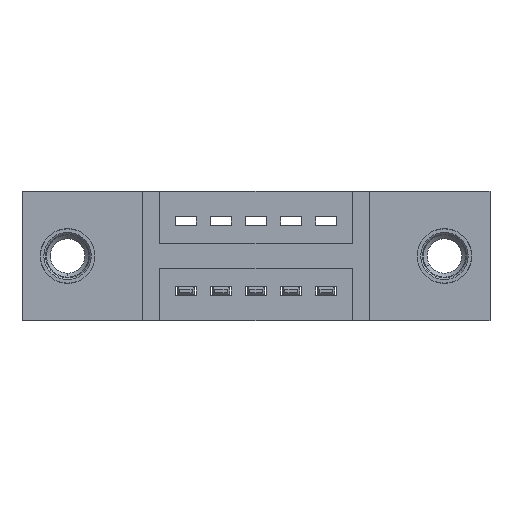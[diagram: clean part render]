
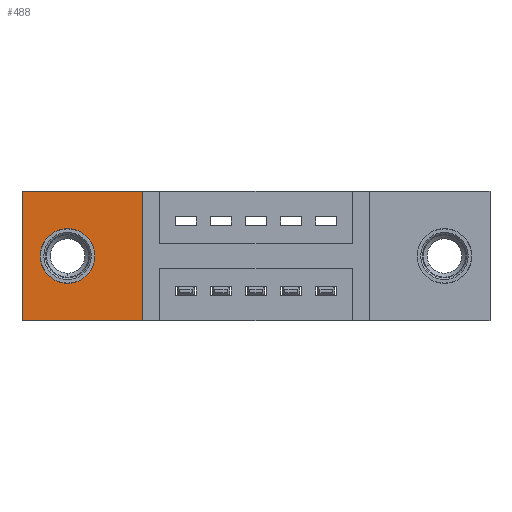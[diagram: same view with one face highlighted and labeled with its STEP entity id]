
A CAD part, front view. The second image highlights one B-rep face of the part: STEP entity #488.
In plain terms, the highlighted planar face has unit normal (0, -1, 0).
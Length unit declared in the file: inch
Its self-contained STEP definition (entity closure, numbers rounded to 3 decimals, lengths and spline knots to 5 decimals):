
#442 = FACE_BOUND ( 'NONE', #9706, .T. ) ;
#488 = ADVANCED_FACE ( 'NONE', ( #442, #2954 ), #3875, .T. ) ;
#566 = LINE ( 'NONE', #5035, #8496 ) ;
#1081 = AXIS2_PLACEMENT_3D ( 'NONE', #4815, #9822, #5535 ) ;
#1098 = CARTESIAN_POINT ( 'NONE',  ( 0.3425, 0.11, -0.37 ) ) ;
#1114 = ORIENTED_EDGE ( 'NONE', *, *, #1237, .T. ) ;
#1181 = CARTESIAN_POINT ( 'NONE',  ( 0.13, 0.11, -0.185 ) ) ;
#1237 = EDGE_CURVE ( 'NONE', #7051, #9205, #566, .T. ) ;
#1371 = EDGE_CURVE ( 'NONE', #5738, #6197, #5918, .T. ) ;
#1994 = DIRECTION ( 'NONE',  ( 0., 0., -1. ) ) ;
#2058 = DIRECTION ( 'NONE',  ( 0., 0., -1. ) ) ;
#2172 = CARTESIAN_POINT ( 'NONE',  ( 0., 0.11, 0. ) ) ;
#2687 = DIRECTION ( 'NONE',  ( 1., 0., 0. ) ) ;
#2844 = EDGE_CURVE ( 'NONE', #2900, #3693, #3410, .T. ) ;
#2900 = VERTEX_POINT ( 'NONE', #3859 ) ;
#2954 = FACE_OUTER_BOUND ( 'NONE', #9757, .T. ) ;
#3065 = DIRECTION ( 'NONE',  ( 0., -1., 0. ) ) ;
#3233 = CARTESIAN_POINT ( 'NONE',  ( 0.13, 0.11, -0.263 ) ) ;
#3410 = LINE ( 'NONE', #2172, #5218 ) ;
#3693 = VERTEX_POINT ( 'NONE', #6074 ) ;
#3859 = CARTESIAN_POINT ( 'NONE',  ( 0.3425, 0.11, 0. ) ) ;
#3875 = PLANE ( 'NONE',  #9088 ) ;
#4003 = CARTESIAN_POINT ( 'NONE',  ( 0., 0.11, -0.37 ) ) ;
#4101 = ORIENTED_EDGE ( 'NONE', *, *, #1371, .F. ) ;
#4141 = CARTESIAN_POINT ( 'NONE',  ( 0., 0.11, 0. ) ) ;
#4257 = VECTOR ( 'NONE', #6540, 39.37008 ) ;
#4375 = CARTESIAN_POINT ( 'NONE',  ( 0.3425, 0.11, 0. ) ) ;
#4726 = AXIS2_PLACEMENT_3D ( 'NONE', #1181, #6629, #2058 ) ;
#4815 = CARTESIAN_POINT ( 'NONE',  ( 0.13, 0.11, -0.185 ) ) ;
#5035 = CARTESIAN_POINT ( 'NONE',  ( 0., 0.11, -0.37 ) ) ;
#5188 = EDGE_CURVE ( 'NONE', #3693, #7051, #6234, .T. ) ;
#5218 = VECTOR ( 'NONE', #8172, 39.37008 ) ;
#5535 = DIRECTION ( 'NONE',  ( 0., 0., -1. ) ) ;
#5725 = EDGE_CURVE ( 'NONE', #6197, #5738, #8796, .T. ) ;
#5738 = VERTEX_POINT ( 'NONE', #3233 ) ;
#5918 = CIRCLE ( 'NONE', #4726, 0.078 ) ;
#6008 = VECTOR ( 'NONE', #9890, 39.37008 ) ;
#6054 = ORIENTED_EDGE ( 'NONE', *, *, #7824, .T. ) ;
#6074 = CARTESIAN_POINT ( 'NONE',  ( 0., 0.11, 0. ) ) ;
#6188 = LINE ( 'NONE', #4375, #4257 ) ;
#6197 = VERTEX_POINT ( 'NONE', #8923 ) ;
#6234 = LINE ( 'NONE', #4141, #6008 ) ;
#6540 = DIRECTION ( 'NONE',  ( 0., 0., 1. ) ) ;
#6629 = DIRECTION ( 'NONE',  ( 0., -1., 0. ) ) ;
#6777 = ORIENTED_EDGE ( 'NONE', *, *, #5725, .F. ) ;
#6999 = ORIENTED_EDGE ( 'NONE', *, *, #2844, .T. ) ;
#7051 = VERTEX_POINT ( 'NONE', #8497 ) ;
#7742 = ORIENTED_EDGE ( 'NONE', *, *, #5188, .T. ) ;
#7824 = EDGE_CURVE ( 'NONE', #9205, #2900, #6188, .T. ) ;
#8172 = DIRECTION ( 'NONE',  ( -1., 0., 0. ) ) ;
#8496 = VECTOR ( 'NONE', #2687, 39.37008 ) ;
#8497 = CARTESIAN_POINT ( 'NONE',  ( 0., 0.11, -0.37 ) ) ;
#8796 = CIRCLE ( 'NONE', #1081, 0.078 ) ;
#8923 = CARTESIAN_POINT ( 'NONE',  ( 0.13, 0.11, -0.107 ) ) ;
#9088 = AXIS2_PLACEMENT_3D ( 'NONE', #4003, #3065, #1994 ) ;
#9205 = VERTEX_POINT ( 'NONE', #1098 ) ;
#9706 = EDGE_LOOP ( 'NONE', ( #6777, #4101 ) ) ;
#9757 = EDGE_LOOP ( 'NONE', ( #7742, #1114, #6054, #6999 ) ) ;
#9822 = DIRECTION ( 'NONE',  ( 0., -1., 0. ) ) ;
#9890 = DIRECTION ( 'NONE',  ( 0., 0., -1. ) ) ;
